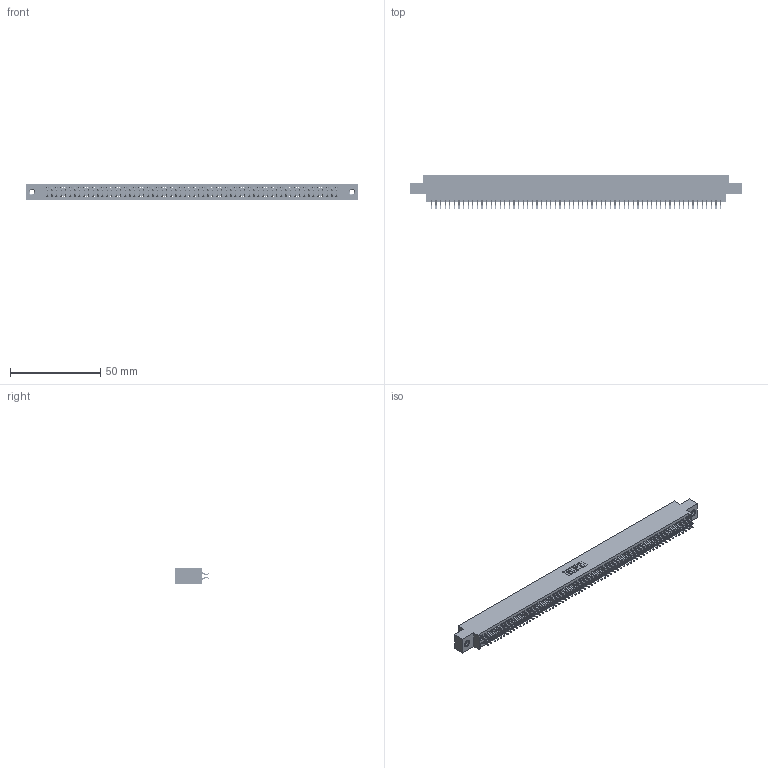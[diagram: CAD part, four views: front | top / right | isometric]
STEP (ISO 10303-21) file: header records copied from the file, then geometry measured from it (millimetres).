
FILE_DESCRIPTION (( 'STEP AP203' ), '1' );
FILE_NAME ('345-128-556-807.STEP', '2018-10-19T21:38:20', ( '' ), ( '' ), 'SwSTEP 2.0', 'SolidWorks 2016', '' );
FILE_SCHEMA (( 'CONFIG_CONTROL_DESIGN' ));
Length unit declared in the file: inch
Products named in the file (4): 345-250-001_345-250-005-103; 345-128-556-807; 345-292-001_556 Tail; 345 Part_0.170 Offset - 0.156 Dia-TI
Assembly tree (131 placements, depth 2):
  345-128-556-807
    345 Part_0.170 Offset - 0.156 Dia-TI
    345-292-001_556 Tail  x128
    345-250-001_345-250-005-103  x2
Bounding box: 183.77 x 19.24 x 9.4 mm (x, y, z)
Volume: 17923.8 mm3; surface area: 26979.7 mm2
Topology: 131 solids, 131 shells, 7358 faces, 21865 edges, 14398 vertices
Faces by surface type: plane 4852, cylinder 2490, cone 12, torus 4
Entity records: 48792 total; most frequent: CARTESIAN_POINT 8155, ORIENTED_EDGE 8070, DIRECTION 7177, EDGE_CURVE 4035, VECTOR 3619, LINE 3619, VERTEX_POINT 2684, AXIS2_PLACEMENT_3D 1779
